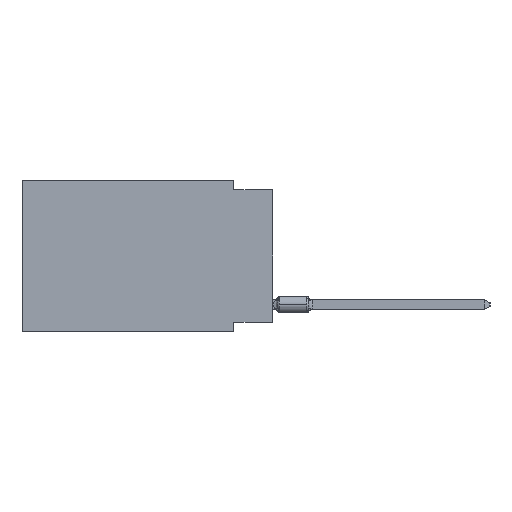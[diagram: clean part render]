
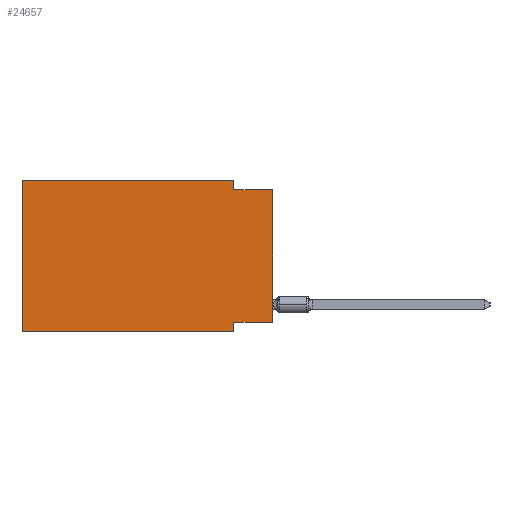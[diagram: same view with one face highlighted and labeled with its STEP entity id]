
A CAD part, left-side view. The second image highlights one B-rep face of the part: STEP entity #24657.
In plain terms, the highlighted planar face has unit normal (-1, 0, 0).
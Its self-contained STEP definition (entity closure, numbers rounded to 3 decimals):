
#479 = CARTESIAN_POINT ( 'NONE',  ( 0., 16.383, -9.906 ) ) ;
#1436 = ORIENTED_EDGE ( 'NONE', *, *, #10591, .F. ) ;
#1679 = CARTESIAN_POINT ( 'NONE',  ( 0., 2.54, -9.906 ) ) ;
#2301 = VECTOR ( 'NONE', #7221, 1000. ) ;
#2494 = DIRECTION ( 'NONE',  ( 0., 0., -1. ) ) ;
#2611 = VERTEX_POINT ( 'NONE', #1679 ) ;
#2890 = VECTOR ( 'NONE', #11568, 1000. ) ;
#3652 = ORIENTED_EDGE ( 'NONE', *, *, #21167, .F. ) ;
#3707 = LINE ( 'NONE', #479, #4376 ) ;
#4038 = CARTESIAN_POINT ( 'NONE',  ( 0., 16.383, 0. ) ) ;
#4293 = DIRECTION ( 'NONE',  ( 0., 0., -1. ) ) ;
#4303 = CARTESIAN_POINT ( 'NONE',  ( 0., 2.54, -9.271 ) ) ;
#4376 = VECTOR ( 'NONE', #23792, 1000. ) ;
#5342 = LINE ( 'NONE', #34507, #9603 ) ;
#5692 = ORIENTED_EDGE ( 'NONE', *, *, #22662, .F. ) ;
#6557 = DIRECTION ( 'NONE',  ( 0., -1., 0. ) ) ;
#7185 = VERTEX_POINT ( 'NONE', #33740 ) ;
#7221 = DIRECTION ( 'NONE',  ( 0., 0., 1. ) ) ;
#7426 = DIRECTION ( 'NONE',  ( 1., 0., 0. ) ) ;
#7448 = VERTEX_POINT ( 'NONE', #32980 ) ;
#7656 = VERTEX_POINT ( 'NONE', #17620 ) ;
#8058 = CARTESIAN_POINT ( 'NONE',  ( 0., 16.383, -9.906 ) ) ;
#8459 = EDGE_CURVE ( 'NONE', #35613, #18920, #12002, .T. ) ;
#9603 = VECTOR ( 'NONE', #2494, 1000. ) ;
#10152 = EDGE_CURVE ( 'NONE', #7185, #18244, #11527, .T. ) ;
#10591 = EDGE_CURVE ( 'NONE', #22777, #7448, #28220, .T. ) ;
#11195 = EDGE_CURVE ( 'NONE', #18244, #2611, #5342, .T. ) ;
#11527 = LINE ( 'NONE', #14789, #2890 ) ;
#11568 = DIRECTION ( 'NONE',  ( 0., 1., 0. ) ) ;
#12002 = LINE ( 'NONE', #12567, #28215 ) ;
#12068 = CARTESIAN_POINT ( 'NONE',  ( 0., 0., -0.635 ) ) ;
#12113 = EDGE_LOOP ( 'NONE', ( #14862, #36130, #5692, #3652, #1436, #20212, #27731, #18432 ) ) ;
#12567 = CARTESIAN_POINT ( 'NONE',  ( 0., 0., -0.635 ) ) ;
#13397 = VECTOR ( 'NONE', #6557, 1000. ) ;
#14315 = LINE ( 'NONE', #32095, #22793 ) ;
#14789 = CARTESIAN_POINT ( 'NONE',  ( 0., 0., -9.271 ) ) ;
#14862 = ORIENTED_EDGE ( 'NONE', *, *, #33945, .T. ) ;
#15796 = FACE_OUTER_BOUND ( 'NONE', #12113, .T. ) ;
#15973 = DIRECTION ( 'NONE',  ( 0., 0., -1. ) ) ;
#16224 = CARTESIAN_POINT ( 'NONE',  ( 0., 2.54, 0. ) ) ;
#17620 = CARTESIAN_POINT ( 'NONE',  ( 0., 2.54, 0. ) ) ;
#18244 = VERTEX_POINT ( 'NONE', #4303 ) ;
#18432 = ORIENTED_EDGE ( 'NONE', *, *, #10152, .F. ) ;
#18905 = EDGE_CURVE ( 'NONE', #22777, #2611, #3707, .T. ) ;
#18920 = VERTEX_POINT ( 'NONE', #12068 ) ;
#20212 = ORIENTED_EDGE ( 'NONE', *, *, #18905, .T. ) ;
#21167 = EDGE_CURVE ( 'NONE', #7448, #7656, #27390, .T. ) ;
#22662 = EDGE_CURVE ( 'NONE', #7656, #35613, #28142, .T. ) ;
#22777 = VERTEX_POINT ( 'NONE', #8058 ) ;
#22793 = VECTOR ( 'NONE', #22823, 1000. ) ;
#22823 = DIRECTION ( 'NONE',  ( 0., 0., 1. ) ) ;
#23792 = DIRECTION ( 'NONE',  ( 0., -1., 0. ) ) ;
#24657 = ADVANCED_FACE ( 'NONE', ( #15796 ), #27163, .F. ) ;
#24824 = CARTESIAN_POINT ( 'NONE',  ( 0., 16.383, 0. ) ) ;
#27133 = DIRECTION ( 'NONE',  ( 0., -1., 0. ) ) ;
#27163 = PLANE ( 'NONE',  #36001 ) ;
#27390 = LINE ( 'NONE', #35893, #13397 ) ;
#27731 = ORIENTED_EDGE ( 'NONE', *, *, #11195, .F. ) ;
#28142 = LINE ( 'NONE', #16224, #35118 ) ;
#28215 = VECTOR ( 'NONE', #27133, 1000. ) ;
#28220 = LINE ( 'NONE', #24824, #2301 ) ;
#32095 = CARTESIAN_POINT ( 'NONE',  ( 0., 0., 0. ) ) ;
#32980 = CARTESIAN_POINT ( 'NONE',  ( 0., 16.383, 0. ) ) ;
#33740 = CARTESIAN_POINT ( 'NONE',  ( 0., 0., -9.271 ) ) ;
#33945 = EDGE_CURVE ( 'NONE', #7185, #18920, #14315, .T. ) ;
#34507 = CARTESIAN_POINT ( 'NONE',  ( 0., 2.54, -9.906 ) ) ;
#35118 = VECTOR ( 'NONE', #4293, 1000. ) ;
#35613 = VERTEX_POINT ( 'NONE', #36510 ) ;
#35893 = CARTESIAN_POINT ( 'NONE',  ( 0., 16.383, 0. ) ) ;
#36001 = AXIS2_PLACEMENT_3D ( 'NONE', #4038, #7426, #15973 ) ;
#36130 = ORIENTED_EDGE ( 'NONE', *, *, #8459, .F. ) ;
#36510 = CARTESIAN_POINT ( 'NONE',  ( 0., 2.54, -0.635 ) ) ;
